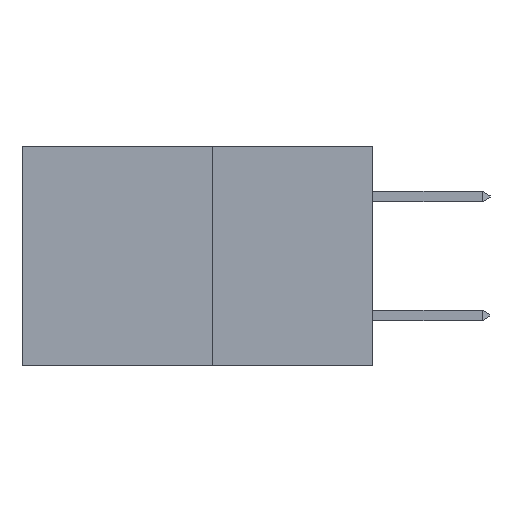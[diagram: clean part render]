
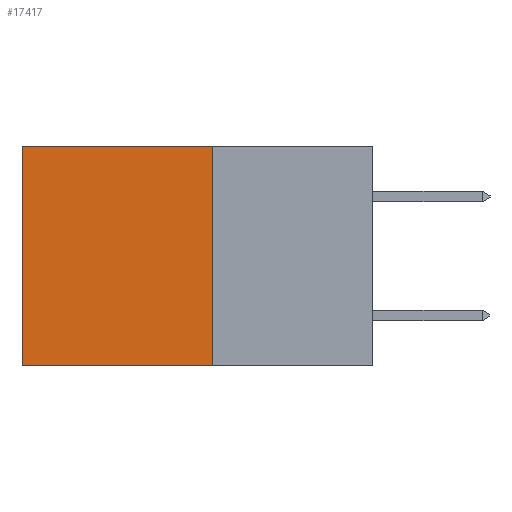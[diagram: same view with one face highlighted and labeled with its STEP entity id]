
A CAD part, left-side view. The second image highlights one B-rep face of the part: STEP entity #17417.
In plain terms, the highlighted planar face has unit normal (-1, 0, 0).
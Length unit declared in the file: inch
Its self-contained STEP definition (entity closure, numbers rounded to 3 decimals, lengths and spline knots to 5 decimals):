
#398 = CARTESIAN_POINT ( 'NONE',  ( 0.277, 0.27, 0. ) ) ;
#537 = CARTESIAN_POINT ( 'NONE',  ( 0.277, 0.59, 0. ) ) ;
#740 = CARTESIAN_POINT ( 'NONE',  ( 0.277, 0.27, -0.37 ) ) ;
#1425 = CARTESIAN_POINT ( 'NONE',  ( 0.277, 0.59, -0.37 ) ) ;
#1787 = LINE ( 'NONE', #3393, #10097 ) ;
#1974 = CARTESIAN_POINT ( 'NONE',  ( 0.277, 0.59, -0.37 ) ) ;
#3393 = CARTESIAN_POINT ( 'NONE',  ( 0.277, 0.27, -0.37 ) ) ;
#4096 = DIRECTION ( 'NONE',  ( 1., 0., 0. ) ) ;
#4301 = VERTEX_POINT ( 'NONE', #9196 ) ;
#4490 = VERTEX_POINT ( 'NONE', #537 ) ;
#5078 = DIRECTION ( 'NONE',  ( 0., 1., 0. ) ) ;
#5737 = CARTESIAN_POINT ( 'NONE',  ( 0.277, 0.27, -0.37 ) ) ;
#6400 = CARTESIAN_POINT ( 'NONE',  ( 0.277, 0.27, -0.37 ) ) ;
#6835 = LINE ( 'NONE', #6400, #13921 ) ;
#7007 = ORIENTED_EDGE ( 'NONE', *, *, #12206, .F. ) ;
#7144 = DIRECTION ( 'NONE',  ( 0., 1., 0. ) ) ;
#7488 = VERTEX_POINT ( 'NONE', #5737 ) ;
#8838 = VECTOR ( 'NONE', #7144, 39.37008 ) ;
#9008 = LINE ( 'NONE', #1974, #12287 ) ;
#9196 = CARTESIAN_POINT ( 'NONE',  ( 0.277, 0.27, 0. ) ) ;
#9649 = AXIS2_PLACEMENT_3D ( 'NONE', #740, #4096, #15484 ) ;
#10097 = VECTOR ( 'NONE', #5078, 39.37008 ) ;
#10690 = PLANE ( 'NONE',  #9649 ) ;
#11349 = EDGE_CURVE ( 'NONE', #4301, #7488, #6835, .T. ) ;
#11896 = DIRECTION ( 'NONE',  ( 0., 0., -1. ) ) ;
#12040 = ORIENTED_EDGE ( 'NONE', *, *, #18524, .T. ) ;
#12206 = EDGE_CURVE ( 'NONE', #7488, #13452, #1787, .T. ) ;
#12252 = ORIENTED_EDGE ( 'NONE', *, *, #14371, .T. ) ;
#12287 = VECTOR ( 'NONE', #11896, 39.37008 ) ;
#13139 = FACE_OUTER_BOUND ( 'NONE', #17365, .T. ) ;
#13452 = VERTEX_POINT ( 'NONE', #1425 ) ;
#13921 = VECTOR ( 'NONE', #19111, 39.37008 ) ;
#14371 = EDGE_CURVE ( 'NONE', #4490, #13452, #9008, .T. ) ;
#15484 = DIRECTION ( 'NONE',  ( 0., 0., -1. ) ) ;
#17365 = EDGE_LOOP ( 'NONE', ( #12252, #7007, #20684, #12040 ) ) ;
#17417 = ADVANCED_FACE ( 'NONE', ( #13139 ), #10690, .F. ) ;
#18524 = EDGE_CURVE ( 'NONE', #4301, #4490, #20857, .T. ) ;
#19111 = DIRECTION ( 'NONE',  ( 0., 0., -1. ) ) ;
#20684 = ORIENTED_EDGE ( 'NONE', *, *, #11349, .F. ) ;
#20857 = LINE ( 'NONE', #398, #8838 ) ;
